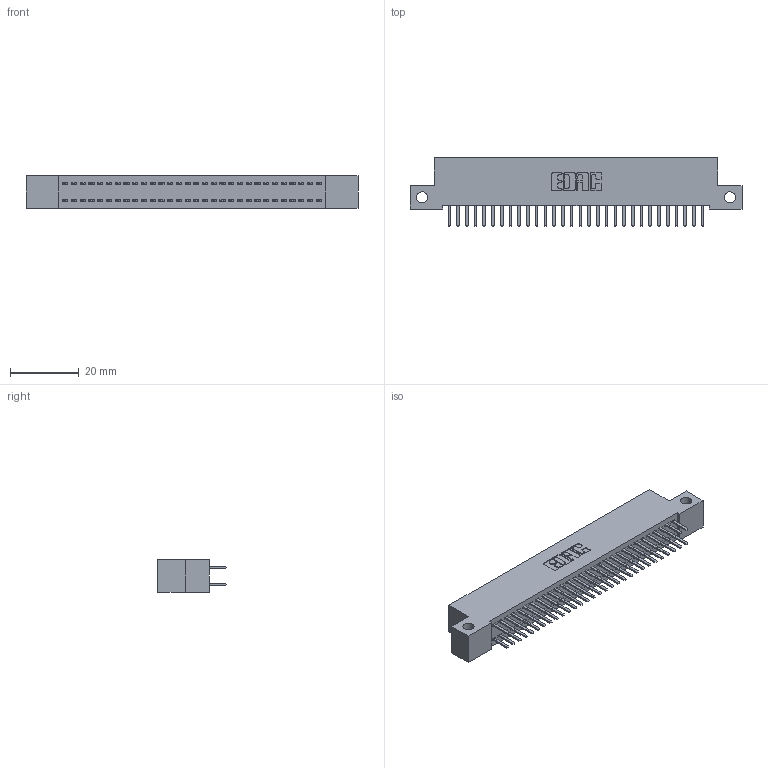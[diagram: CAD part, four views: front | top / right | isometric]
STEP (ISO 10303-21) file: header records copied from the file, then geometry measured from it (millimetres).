
FILE_DESCRIPTION (( 'STEP AP203' ), '1' );
FILE_NAME ('342-060-520-212.STEP', '2018-08-13T05:58:04', ( '' ), ( '' ), 'SwSTEP 2.0', 'SolidWorks 2016', '' );
FILE_SCHEMA (( 'CONFIG_CONTROL_DESIGN' ));
Length unit declared in the file: inch
Products named in the file (3): 342 Part_Side Mount; 345-292-001_345-293-120; 342-060-520-212
Assembly tree (61 placements, depth 2):
  342-060-520-212
    342 Part_Side Mount
    345-292-001_345-293-120  x60
Bounding box: 96.52 x 20.02 x 9.4 mm (x, y, z)
Volume: 8515.2 mm3; surface area: 13342.9 mm2
Topology: 61 solids, 61 shells, 3470 faces, 10079 edges, 6558 vertices
Faces by surface type: plane 2346, cylinder 1124
Entity records: 20837 total; most frequent: CARTESIAN_POINT 3478, ORIENTED_EDGE 3402, DIRECTION 2981, EDGE_CURVE 1701, LINE 1569, VECTOR 1569, VERTEX_POINT 1130, AXIS2_PLACEMENT_3D 706
